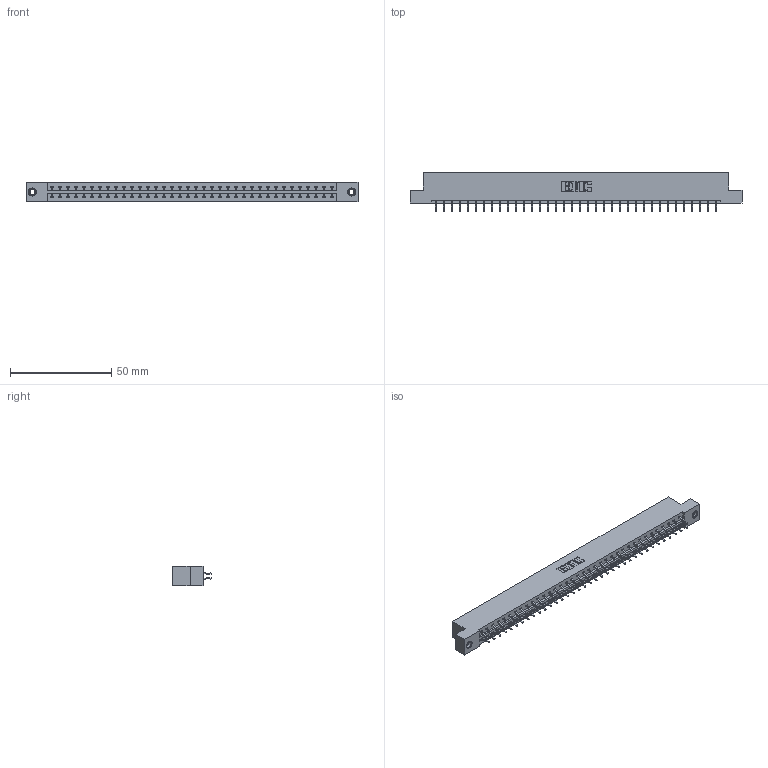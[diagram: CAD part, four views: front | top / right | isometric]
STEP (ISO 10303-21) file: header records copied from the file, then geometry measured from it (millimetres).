
FILE_DESCRIPTION (( 'STEP AP203' ), '1' );
FILE_NAME ('833-072-556-207.STEP', '2020-06-05T14:51:42', ( '' ), ( '' ), 'SwSTEP 2.0', 'SolidWorks 2020', '' );
FILE_SCHEMA (( 'CONFIG_CONTROL_DESIGN' ));
Length unit declared in the file: inch
Products named in the file (4): 345-292-001_556 Tail; 833-072-556-207; 833 Part_Flush - .156 Dia - TI; 345-250-001_345-250-005-103
Assembly tree (75 placements, depth 2):
  833-072-556-207
    833 Part_Flush - .156 Dia - TI
    345-292-001_556 Tail  x72
    345-250-001_345-250-005-103  x2
Bounding box: 164.19 x 19.57 x 9.4 mm (x, y, z)
Volume: 16689.9 mm3; surface area: 19630.3 mm2
Topology: 75 solids, 75 shells, 4350 faces, 12903 edges, 8498 vertices
Faces by surface type: plane 2982, cylinder 1352, cone 12, torus 4
Entity records: 25342 total; most frequent: CARTESIAN_POINT 4205, ORIENTED_EDGE 4122, DIRECTION 3623, EDGE_CURVE 2061, VECTOR 1905, LINE 1905, VERTEX_POINT 1368, AXIS2_PLACEMENT_3D 859
